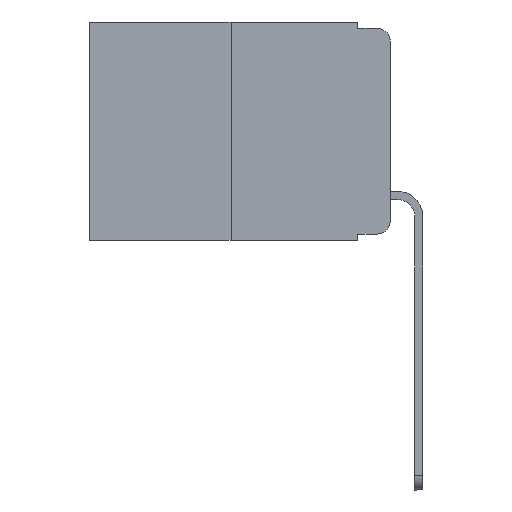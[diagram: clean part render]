
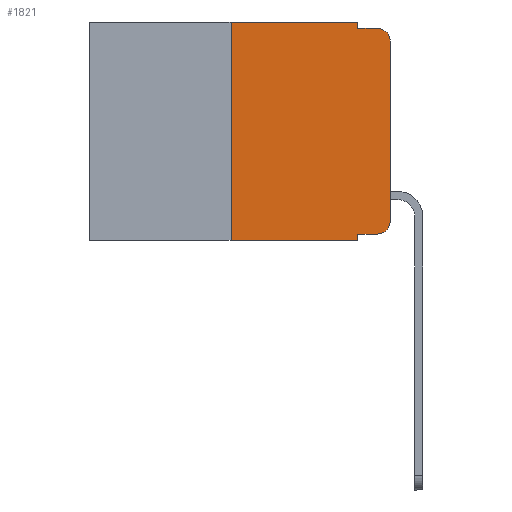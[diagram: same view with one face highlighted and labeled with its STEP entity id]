
A CAD part, left-side view. The second image highlights one B-rep face of the part: STEP entity #1821.
In plain terms, the highlighted planar face has unit normal (-1, 0, 0).
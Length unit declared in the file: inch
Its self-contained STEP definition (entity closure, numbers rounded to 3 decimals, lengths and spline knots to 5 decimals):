
#83 = ORIENTED_EDGE ( 'NONE', *, *, #7894, .T. ) ;
#139 = ORIENTED_EDGE ( 'NONE', *, *, #7073, .F. ) ;
#246 = VECTOR ( 'NONE', #2664, 39.37008 ) ;
#411 = CARTESIAN_POINT ( 'NONE',  ( 0., 0.473, -0.343 ) ) ;
#544 = VERTEX_POINT ( 'NONE', #6132 ) ;
#770 = ORIENTED_EDGE ( 'NONE', *, *, #8896, .F. ) ;
#839 = DIRECTION ( 'NONE',  ( 0., -1., 0. ) ) ;
#893 = ORIENTED_EDGE ( 'NONE', *, *, #9997, .T. ) ;
#1512 = CARTESIAN_POINT ( 'NONE',  ( 0., 0.473, 0. ) ) ;
#1584 = CARTESIAN_POINT ( 'NONE',  ( 0., 0.02, -0.03 ) ) ;
#1642 = CARTESIAN_POINT ( 'NONE',  ( 0., 0.051, 0. ) ) ;
#1738 = LINE ( 'NONE', #1642, #12037 ) ;
#1811 = CARTESIAN_POINT ( 'NONE',  ( 0., 0.02, -0.01 ) ) ;
#1821 = ADVANCED_FACE ( 'NONE', ( #5473 ), #2732, .F. ) ;
#2085 = DIRECTION ( 'NONE',  ( -1., 0., 0. ) ) ;
#2128 = VERTEX_POINT ( 'NONE', #11455 ) ;
#2219 = CARTESIAN_POINT ( 'NONE',  ( 0., 0.02, -0.313 ) ) ;
#2242 = DIRECTION ( 'NONE',  ( 0., 0., -1. ) ) ;
#2325 = EDGE_CURVE ( 'NONE', #5049, #6136, #12781, .T. ) ;
#2482 = EDGE_LOOP ( 'NONE', ( #83, #2958, #4600, #139, #770, #3273, #893, #3332, #3186, #7134 ) ) ;
#2663 = DIRECTION ( 'NONE',  ( 0., 0., -1. ) ) ;
#2664 = DIRECTION ( 'NONE',  ( 0., -1., 0. ) ) ;
#2732 = PLANE ( 'NONE',  #2875 ) ;
#2773 = CARTESIAN_POINT ( 'NONE',  ( 0., 0.051, -0.01 ) ) ;
#2875 = AXIS2_PLACEMENT_3D ( 'NONE', #1512, #3139, #8807 ) ;
#2901 = CARTESIAN_POINT ( 'NONE',  ( 0., 0., -0.03 ) ) ;
#2958 = ORIENTED_EDGE ( 'NONE', *, *, #6904, .T. ) ;
#3027 = CARTESIAN_POINT ( 'NONE',  ( 0., 0.473, 0. ) ) ;
#3139 = DIRECTION ( 'NONE',  ( 1., 0., 0. ) ) ;
#3186 = ORIENTED_EDGE ( 'NONE', *, *, #11879, .T. ) ;
#3273 = ORIENTED_EDGE ( 'NONE', *, *, #3724, .F. ) ;
#3288 = VERTEX_POINT ( 'NONE', #1811 ) ;
#3332 = ORIENTED_EDGE ( 'NONE', *, *, #10591, .F. ) ;
#3490 = LINE ( 'NONE', #7203, #8544 ) ;
#3592 = VECTOR ( 'NONE', #8634, 39.37008 ) ;
#3613 = DIRECTION ( 'NONE',  ( 0., -1., 0. ) ) ;
#3711 = DIRECTION ( 'NONE',  ( 0., 0., 1. ) ) ;
#3724 = EDGE_CURVE ( 'NONE', #2128, #7414, #3490, .T. ) ;
#4250 = CARTESIAN_POINT ( 'NONE',  ( 0., 0.02, -0.333 ) ) ;
#4500 = VECTOR ( 'NONE', #3613, 39.37008 ) ;
#4600 = ORIENTED_EDGE ( 'NONE', *, *, #9506, .F. ) ;
#5049 = VERTEX_POINT ( 'NONE', #4250 ) ;
#5094 = VECTOR ( 'NONE', #839, 39.37008 ) ;
#5309 = CARTESIAN_POINT ( 'NONE',  ( 0., 0.25, 0. ) ) ;
#5404 = LINE ( 'NONE', #3027, #5094 ) ;
#5473 = FACE_OUTER_BOUND ( 'NONE', #2482, .T. ) ;
#6132 = CARTESIAN_POINT ( 'NONE',  ( 0., 0.051, -0.333 ) ) ;
#6136 = VERTEX_POINT ( 'NONE', #10721 ) ;
#6363 = CIRCLE ( 'NONE', #12719, 0.02 ) ;
#6904 = EDGE_CURVE ( 'NONE', #12126, #3288, #6363, .T. ) ;
#7073 = EDGE_CURVE ( 'NONE', #10750, #7578, #1738, .T. ) ;
#7134 = ORIENTED_EDGE ( 'NONE', *, *, #2325, .T. ) ;
#7203 = CARTESIAN_POINT ( 'NONE',  ( 0., 0.25, 0. ) ) ;
#7414 = VERTEX_POINT ( 'NONE', #5309 ) ;
#7578 = VERTEX_POINT ( 'NONE', #12372 ) ;
#7644 = CARTESIAN_POINT ( 'NONE',  ( 0., 0.051, 0. ) ) ;
#7894 = EDGE_CURVE ( 'NONE', #6136, #12126, #8242, .T. ) ;
#8242 = LINE ( 'NONE', #9802, #12164 ) ;
#8544 = VECTOR ( 'NONE', #3711, 39.37008 ) ;
#8634 = DIRECTION ( 'NONE',  ( 0., 0., -1. ) ) ;
#8652 = CARTESIAN_POINT ( 'NONE',  ( 0., 0.051, -0.333 ) ) ;
#8666 = VERTEX_POINT ( 'NONE', #9738 ) ;
#8672 = DIRECTION ( 'NONE',  ( -1., 0., 0. ) ) ;
#8729 = DIRECTION ( 'NONE',  ( 0., 0., -1. ) ) ;
#8807 = DIRECTION ( 'NONE',  ( 0., 0., -1. ) ) ;
#8896 = EDGE_CURVE ( 'NONE', #7414, #10750, #5404, .T. ) ;
#9410 = LINE ( 'NONE', #2773, #9722 ) ;
#9506 = EDGE_CURVE ( 'NONE', #7578, #3288, #9410, .T. ) ;
#9722 = VECTOR ( 'NONE', #12583, 39.37008 ) ;
#9738 = CARTESIAN_POINT ( 'NONE',  ( 0., 0.051, -0.343 ) ) ;
#9800 = CARTESIAN_POINT ( 'NONE',  ( 0., 0.051, 0. ) ) ;
#9802 = CARTESIAN_POINT ( 'NONE',  ( 0., 0., 0. ) ) ;
#9997 = EDGE_CURVE ( 'NONE', #2128, #8666, #11091, .T. ) ;
#10591 = EDGE_CURVE ( 'NONE', #544, #8666, #11528, .T. ) ;
#10620 = AXIS2_PLACEMENT_3D ( 'NONE', #2219, #2085, #2242 ) ;
#10721 = CARTESIAN_POINT ( 'NONE',  ( 0., 0., -0.313 ) ) ;
#10750 = VERTEX_POINT ( 'NONE', #9800 ) ;
#11091 = LINE ( 'NONE', #411, #246 ) ;
#11455 = CARTESIAN_POINT ( 'NONE',  ( 0., 0.25, -0.343 ) ) ;
#11528 = LINE ( 'NONE', #7644, #3592 ) ;
#11879 = EDGE_CURVE ( 'NONE', #544, #5049, #12349, .T. ) ;
#12037 = VECTOR ( 'NONE', #8729, 39.37008 ) ;
#12126 = VERTEX_POINT ( 'NONE', #2901 ) ;
#12164 = VECTOR ( 'NONE', #12692, 39.37008 ) ;
#12349 = LINE ( 'NONE', #8652, #4500 ) ;
#12372 = CARTESIAN_POINT ( 'NONE',  ( 0., 0.051, -0.01 ) ) ;
#12583 = DIRECTION ( 'NONE',  ( 0., -1., 0. ) ) ;
#12692 = DIRECTION ( 'NONE',  ( 0., 0., 1. ) ) ;
#12719 = AXIS2_PLACEMENT_3D ( 'NONE', #1584, #8672, #2663 ) ;
#12781 = CIRCLE ( 'NONE', #10620, 0.02 ) ;
